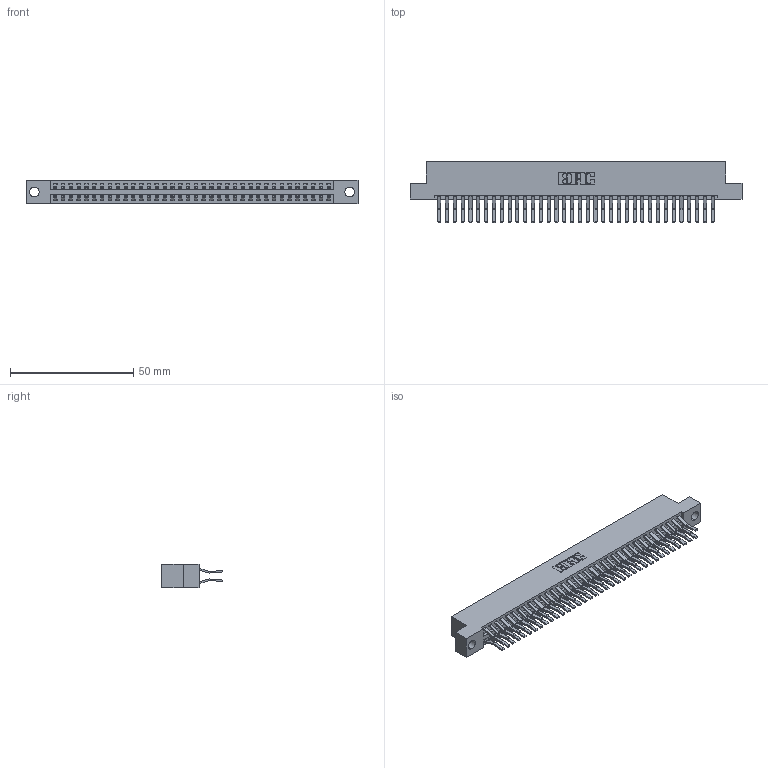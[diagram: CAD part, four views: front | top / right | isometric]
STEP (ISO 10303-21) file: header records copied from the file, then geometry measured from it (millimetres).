
FILE_DESCRIPTION (( 'STEP AP203' ), '1' );
FILE_NAME ('396-072-560-204.STEP', '2018-09-09T11:07:15', ( '' ), ( '' ), 'SwSTEP 2.0', 'SolidWorks 2016', '' );
FILE_SCHEMA (( 'CONFIG_CONTROL_DESIGN' ));
Length unit declared in the file: inch
Products named in the file (3): 396-072-560-204; 346 Part_Flush Mounting Lugs - 0.156 Dia-TH; 345-292-001_560 Tail
Assembly tree (73 placements, depth 2):
  396-072-560-204
    346 Part_Flush Mounting Lugs - 0.156 Dia-TH
    345-292-001_560 Tail  x72
Bounding box: 134.87 x 24.78 x 9.4 mm (x, y, z)
Volume: 13489.4 mm3; surface area: 19520.2 mm2
Topology: 73 solids, 73 shells, 4010 faces, 11921 edges, 7850 vertices
Faces by surface type: plane 2596, cylinder 1414
Entity records: 24393 total; most frequent: CARTESIAN_POINT 4028, ORIENTED_EDGE 3962, DIRECTION 3605, EDGE_CURVE 1981, LINE 1701, VECTOR 1701, VERTEX_POINT 1318, AXIS2_PLACEMENT_3D 952
